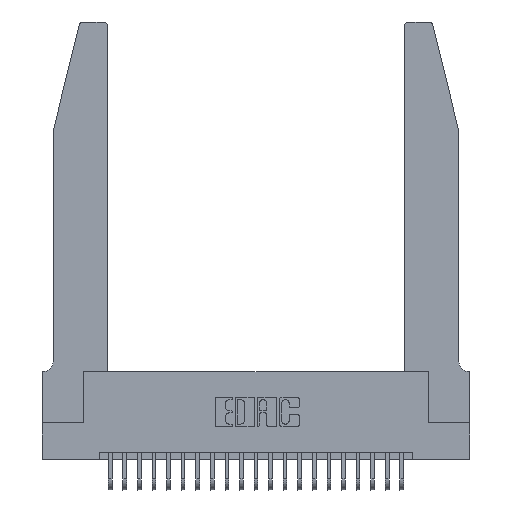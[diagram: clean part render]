
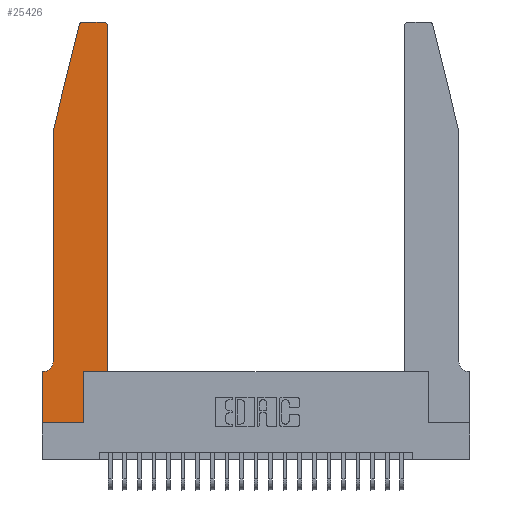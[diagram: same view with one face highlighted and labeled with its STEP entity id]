
A CAD part, top view. The second image highlights one B-rep face of the part: STEP entity #25426.
In plain terms, the highlighted planar face has unit normal (0, 0, 1).
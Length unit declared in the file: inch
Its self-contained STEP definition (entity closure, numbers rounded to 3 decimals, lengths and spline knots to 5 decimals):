
#80 = EDGE_CURVE ( 'NONE', #14567, #25148, #841, .T. ) ;
#439 = ORIENTED_EDGE ( 'NONE', *, *, #8306, .T. ) ;
#483 = ORIENTED_EDGE ( 'NONE', *, *, #11313, .T. ) ;
#841 = CIRCLE ( 'NONE', #16332, 0.07 ) ;
#884 = VERTEX_POINT ( 'NONE', #2227 ) ;
#923 = VERTEX_POINT ( 'NONE', #10475 ) ;
#981 = EDGE_CURVE ( 'NONE', #923, #7402, #4837, .T. ) ;
#1335 = CARTESIAN_POINT ( 'NONE',  ( 0.25487, 2.72718, 0.37 ) ) ;
#1516 = LINE ( 'NONE', #19575, #16714 ) ;
#1620 = ORIENTED_EDGE ( 'NONE', *, *, #981, .T. ) ;
#2227 = CARTESIAN_POINT ( 'NONE',  ( 0.2865, 0., 0.37 ) ) ;
#2437 = DIRECTION ( 'NONE',  ( -1., 0., 0. ) ) ;
#2546 = LINE ( 'NONE', #15064, #7814 ) ;
#2672 = CARTESIAN_POINT ( 'NONE',  ( 0., 0.35, 0.37 ) ) ;
#2833 = CARTESIAN_POINT ( 'NONE',  ( 0.0755, 2., 0.37 ) ) ;
#3243 = CARTESIAN_POINT ( 'NONE',  ( 0., 0., 0.37 ) ) ;
#3491 = DIRECTION ( 'NONE',  ( 0., -1., 0. ) ) ;
#3533 = CARTESIAN_POINT ( 'NONE',  ( 0.4505, 0.35, 0.37 ) ) ;
#3598 = CARTESIAN_POINT ( 'NONE',  ( 0.0055, 0.35, 0.37 ) ) ;
#4460 = EDGE_CURVE ( 'NONE', #7402, #17114, #2546, .T. ) ;
#4476 = VERTEX_POINT ( 'NONE', #3243 ) ;
#4618 = DIRECTION ( 'NONE',  ( 1., 0., 0. ) ) ;
#4785 = VECTOR ( 'NONE', #8334, 39.37008 ) ;
#4837 = CIRCLE ( 'NONE', #12188, 0.03 ) ;
#5143 = AXIS2_PLACEMENT_3D ( 'NONE', #8411, #12409, #12580 ) ;
#5521 = ORIENTED_EDGE ( 'NONE', *, *, #20417, .T. ) ;
#6221 = VERTEX_POINT ( 'NONE', #20628 ) ;
#6482 = LINE ( 'NONE', #15578, #12069 ) ;
#6635 = EDGE_CURVE ( 'NONE', #25148, #8311, #6482, .T. ) ;
#7255 = DIRECTION ( 'NONE',  ( 0., -1., 0. ) ) ;
#7402 = VERTEX_POINT ( 'NONE', #1335 ) ;
#7407 = EDGE_CURVE ( 'NONE', #19077, #923, #1516, .T. ) ;
#7476 = EDGE_CURVE ( 'NONE', #17114, #14567, #10797, .T. ) ;
#7788 = ORIENTED_EDGE ( 'NONE', *, *, #6635, .T. ) ;
#7814 = VECTOR ( 'NONE', #17091, 39.37008 ) ;
#7975 = CIRCLE ( 'NONE', #5143, 0.03 ) ;
#8306 = EDGE_CURVE ( 'NONE', #17652, #19077, #7975, .T. ) ;
#8311 = VERTEX_POINT ( 'NONE', #2672 ) ;
#8334 = DIRECTION ( 'NONE',  ( 0., 1., 0. ) ) ;
#8337 = VECTOR ( 'NONE', #23646, 39.37008 ) ;
#8385 = DIRECTION ( 'NONE',  ( 0., 0., 1. ) ) ;
#8411 = CARTESIAN_POINT ( 'NONE',  ( 0.4205, 2.72, 0.37 ) ) ;
#8430 = ORIENTED_EDGE ( 'NONE', *, *, #80, .T. ) ;
#8554 = VERTEX_POINT ( 'NONE', #15665 ) ;
#9121 = LINE ( 'NONE', #24155, #22491 ) ;
#10064 = DIRECTION ( 'NONE',  ( 1., 0., 0. ) ) ;
#10475 = CARTESIAN_POINT ( 'NONE',  ( 0.284, 2.75, 0.37 ) ) ;
#10501 = LINE ( 'NONE', #20943, #8337 ) ;
#10797 = LINE ( 'NONE', #19392, #11417 ) ;
#11313 = EDGE_CURVE ( 'NONE', #8554, #6221, #11538, .T. ) ;
#11417 = VECTOR ( 'NONE', #3491, 39.37008 ) ;
#11456 = DIRECTION ( 'NONE',  ( 1., 0., 0. ) ) ;
#11538 = LINE ( 'NONE', #3533, #16198 ) ;
#11869 = ORIENTED_EDGE ( 'NONE', *, *, #7476, .T. ) ;
#12069 = VECTOR ( 'NONE', #19148, 39.37008 ) ;
#12093 = ORIENTED_EDGE ( 'NONE', *, *, #18289, .T. ) ;
#12188 = AXIS2_PLACEMENT_3D ( 'NONE', #18713, #24440, #4618 ) ;
#12329 = CARTESIAN_POINT ( 'NONE',  ( 0.2865, 0.35, 0.37 ) ) ;
#12409 = DIRECTION ( 'NONE',  ( 0., 0., 1. ) ) ;
#12580 = DIRECTION ( 'NONE',  ( 1., 0., 0. ) ) ;
#14016 = CARTESIAN_POINT ( 'NONE',  ( 0.4505, 2.72, 0.37 ) ) ;
#14026 = VECTOR ( 'NONE', #7255, 39.37008 ) ;
#14345 = LINE ( 'NONE', #21247, #14026 ) ;
#14567 = VERTEX_POINT ( 'NONE', #17170 ) ;
#15019 = AXIS2_PLACEMENT_3D ( 'NONE', #20281, #8385, #22292 ) ;
#15064 = CARTESIAN_POINT ( 'NONE',  ( 0.0755, 2., 0.37 ) ) ;
#15578 = CARTESIAN_POINT ( 'NONE',  ( 0.0755, 0.35, 0.37 ) ) ;
#15665 = CARTESIAN_POINT ( 'NONE',  ( 0.2865, 0.35, 0.37 ) ) ;
#16026 = EDGE_CURVE ( 'NONE', #6221, #17652, #10501, .T. ) ;
#16198 = VECTOR ( 'NONE', #11456, 39.37008 ) ;
#16332 = AXIS2_PLACEMENT_3D ( 'NONE', #24250, #24333, #2437 ) ;
#16704 = CARTESIAN_POINT ( 'NONE',  ( 0.4205, 2.75, 0.37 ) ) ;
#16714 = VECTOR ( 'NONE', #23421, 39.37008 ) ;
#17091 = DIRECTION ( 'NONE',  ( -0.239, -0.971, 0. ) ) ;
#17114 = VERTEX_POINT ( 'NONE', #2833 ) ;
#17170 = CARTESIAN_POINT ( 'NONE',  ( 0.0755, 0.42, 0.37 ) ) ;
#17480 = FACE_OUTER_BOUND ( 'NONE', #22430, .T. ) ;
#17652 = VERTEX_POINT ( 'NONE', #14016 ) ;
#18289 = EDGE_CURVE ( 'NONE', #884, #8554, #23782, .T. ) ;
#18713 = CARTESIAN_POINT ( 'NONE',  ( 0.284, 2.72, 0.37 ) ) ;
#18721 = ORIENTED_EDGE ( 'NONE', *, *, #7407, .T. ) ;
#19077 = VERTEX_POINT ( 'NONE', #16704 ) ;
#19148 = DIRECTION ( 'NONE',  ( -1., 0., 0. ) ) ;
#19392 = CARTESIAN_POINT ( 'NONE',  ( 0.0755, 2., 0.37 ) ) ;
#19485 = EDGE_CURVE ( 'NONE', #4476, #884, #9121, .T. ) ;
#19575 = CARTESIAN_POINT ( 'NONE',  ( 0.2605, 2.75, 0.37 ) ) ;
#20281 = CARTESIAN_POINT ( 'NONE',  ( 0., 0.35, 0.37 ) ) ;
#20417 = EDGE_CURVE ( 'NONE', #8311, #4476, #14345, .T. ) ;
#20628 = CARTESIAN_POINT ( 'NONE',  ( 0.4505, 0.35, 0.37 ) ) ;
#20943 = CARTESIAN_POINT ( 'NONE',  ( 0.4505, 0.35, 0.37 ) ) ;
#21247 = CARTESIAN_POINT ( 'NONE',  ( 0., 0., 0.37 ) ) ;
#21945 = PLANE ( 'NONE',  #15019 ) ;
#21978 = ORIENTED_EDGE ( 'NONE', *, *, #19485, .T. ) ;
#22292 = DIRECTION ( 'NONE',  ( 1., 0., 0. ) ) ;
#22430 = EDGE_LOOP ( 'NONE', ( #18721, #1620, #25573, #11869, #8430, #7788, #5521, #21978, #12093, #483, #23490, #439 ) ) ;
#22491 = VECTOR ( 'NONE', #10064, 39.37008 ) ;
#23421 = DIRECTION ( 'NONE',  ( -1., 0., 0. ) ) ;
#23490 = ORIENTED_EDGE ( 'NONE', *, *, #16026, .T. ) ;
#23646 = DIRECTION ( 'NONE',  ( 0., 1., 0. ) ) ;
#23782 = LINE ( 'NONE', #12329, #4785 ) ;
#24155 = CARTESIAN_POINT ( 'NONE',  ( 0., 0., 0.37 ) ) ;
#24250 = CARTESIAN_POINT ( 'NONE',  ( 0.0055, 0.42, 0.37 ) ) ;
#24333 = DIRECTION ( 'NONE',  ( 0., 0., -1. ) ) ;
#24440 = DIRECTION ( 'NONE',  ( 0., 0., 1. ) ) ;
#25148 = VERTEX_POINT ( 'NONE', #3598 ) ;
#25426 = ADVANCED_FACE ( 'NONE', ( #17480 ), #21945, .T. ) ;
#25573 = ORIENTED_EDGE ( 'NONE', *, *, #4460, .T. ) ;
